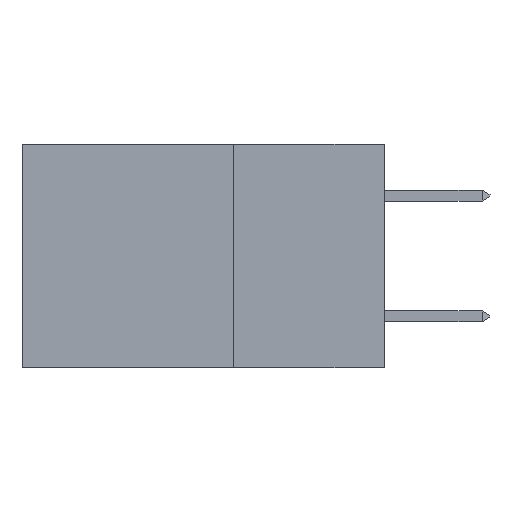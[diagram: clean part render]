
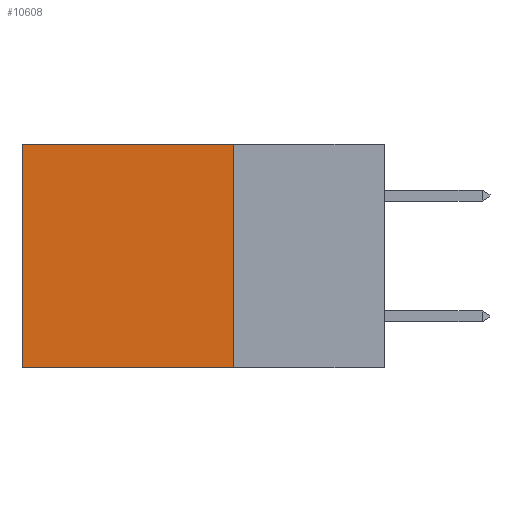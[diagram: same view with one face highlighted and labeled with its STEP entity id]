
A CAD part, left-side view. The second image highlights one B-rep face of the part: STEP entity #10608.
In plain terms, the highlighted planar face has unit normal (-1, 0, 0).
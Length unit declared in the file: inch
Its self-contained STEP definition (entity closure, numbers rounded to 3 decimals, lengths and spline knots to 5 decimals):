
#866 = VERTEX_POINT ( 'NONE', #17377 ) ;
#1686 = VECTOR ( 'NONE', #16259, 39.37008 ) ;
#2469 = CARTESIAN_POINT ( 'NONE',  ( 0.2875, 0.25, 0. ) ) ;
#3050 = ORIENTED_EDGE ( 'NONE', *, *, #5797, .F. ) ;
#5371 = VECTOR ( 'NONE', #16469, 39.37008 ) ;
#5797 = EDGE_CURVE ( 'NONE', #23247, #16277, #24258, .T. ) ;
#6886 = CARTESIAN_POINT ( 'NONE',  ( 0.2875, 0.25, 0. ) ) ;
#7079 = LINE ( 'NONE', #14350, #1686 ) ;
#7298 = LINE ( 'NONE', #25050, #13234 ) ;
#8323 = VECTOR ( 'NONE', #16113, 39.37008 ) ;
#10608 = ADVANCED_FACE ( 'NONE', ( #11193 ), #22750, .F. ) ;
#11140 = DIRECTION ( 'NONE',  ( 0., 0., -1. ) ) ;
#11193 = FACE_OUTER_BOUND ( 'NONE', #11973, .T. ) ;
#11309 = LINE ( 'NONE', #2469, #5371 ) ;
#11973 = EDGE_LOOP ( 'NONE', ( #18930, #21275, #3050, #16253 ) ) ;
#12288 = VERTEX_POINT ( 'NONE', #16562 ) ;
#12883 = DIRECTION ( 'NONE',  ( 0., 0., -1. ) ) ;
#13234 = VECTOR ( 'NONE', #11140, 39.37008 ) ;
#13706 = CARTESIAN_POINT ( 'NONE',  ( 0.2875, 0.25, 0. ) ) ;
#14249 = EDGE_CURVE ( 'NONE', #23247, #12288, #11309, .T. ) ;
#14350 = CARTESIAN_POINT ( 'NONE',  ( 0.2875, 0.25, -0.37 ) ) ;
#14784 = AXIS2_PLACEMENT_3D ( 'NONE', #20825, #24779, #12883 ) ;
#16113 = DIRECTION ( 'NONE',  ( 0., 0., -1. ) ) ;
#16253 = ORIENTED_EDGE ( 'NONE', *, *, #14249, .T. ) ;
#16259 = DIRECTION ( 'NONE',  ( 0., 1., 0. ) ) ;
#16277 = VERTEX_POINT ( 'NONE', #20972 ) ;
#16469 = DIRECTION ( 'NONE',  ( 0., 1., 0. ) ) ;
#16562 = CARTESIAN_POINT ( 'NONE',  ( 0.2875, 0.6, 0. ) ) ;
#17377 = CARTESIAN_POINT ( 'NONE',  ( 0.2875, 0.6, -0.37 ) ) ;
#18930 = ORIENTED_EDGE ( 'NONE', *, *, #23352, .T. ) ;
#20825 = CARTESIAN_POINT ( 'NONE',  ( 0.2875, 0.25, 0. ) ) ;
#20972 = CARTESIAN_POINT ( 'NONE',  ( 0.2875, 0.25, -0.37 ) ) ;
#21275 = ORIENTED_EDGE ( 'NONE', *, *, #21798, .F. ) ;
#21798 = EDGE_CURVE ( 'NONE', #16277, #866, #7079, .T. ) ;
#22750 = PLANE ( 'NONE',  #14784 ) ;
#23247 = VERTEX_POINT ( 'NONE', #6886 ) ;
#23352 = EDGE_CURVE ( 'NONE', #12288, #866, #7298, .T. ) ;
#24258 = LINE ( 'NONE', #13706, #8323 ) ;
#24779 = DIRECTION ( 'NONE',  ( 1., 0., 0. ) ) ;
#25050 = CARTESIAN_POINT ( 'NONE',  ( 0.2875, 0.6, 0. ) ) ;
